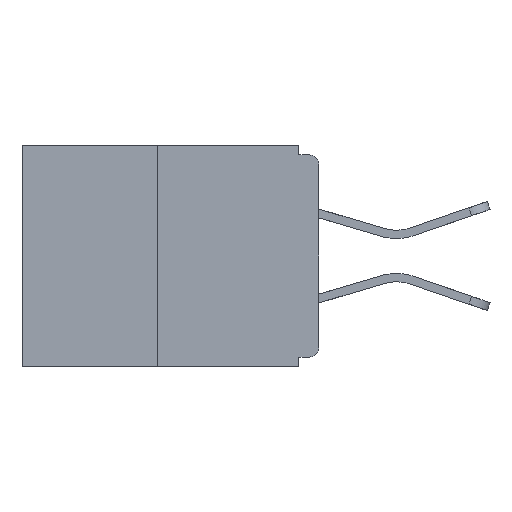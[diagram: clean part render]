
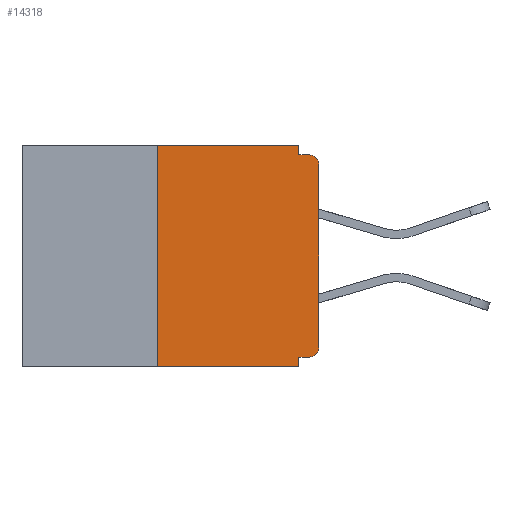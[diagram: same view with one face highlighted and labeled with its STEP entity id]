
A CAD part, left-side view. The second image highlights one B-rep face of the part: STEP entity #14318.
In plain terms, the highlighted planar face has unit normal (-1, 0, 0).
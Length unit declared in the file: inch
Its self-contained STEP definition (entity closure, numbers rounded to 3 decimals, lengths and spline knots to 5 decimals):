
#221 = PLANE ( 'NONE',  #11484 ) ;
#330 = DIRECTION ( 'NONE',  ( 0., 0., 1. ) ) ;
#594 = VERTEX_POINT ( 'NONE', #8248 ) ;
#719 = EDGE_LOOP ( 'NONE', ( #12575, #25406, #7802, #6723, #24492, #20611, #23564, #11362, #3248, #17616 ) ) ;
#834 = DIRECTION ( 'NONE',  ( 0., 0., -1. ) ) ;
#913 = CARTESIAN_POINT ( 'NONE',  ( 0., 0.031, -0.343 ) ) ;
#1100 = CARTESIAN_POINT ( 'NONE',  ( 0., 0., -0.03 ) ) ;
#1107 = DIRECTION ( 'NONE',  ( -1., 0., 0. ) ) ;
#1540 = AXIS2_PLACEMENT_3D ( 'NONE', #4196, #25913, #23711 ) ;
#1743 = FACE_OUTER_BOUND ( 'NONE', #719, .T. ) ;
#1822 = VERTEX_POINT ( 'NONE', #11964 ) ;
#2160 = DIRECTION ( 'NONE',  ( 0., 0., -1. ) ) ;
#2298 = VECTOR ( 'NONE', #2160, 39.37008 ) ;
#2478 = CARTESIAN_POINT ( 'NONE',  ( 0., 0., 0. ) ) ;
#3248 = ORIENTED_EDGE ( 'NONE', *, *, #22744, .F. ) ;
#3384 = VERTEX_POINT ( 'NONE', #913 ) ;
#3580 = VECTOR ( 'NONE', #10918, 39.37008 ) ;
#4196 = CARTESIAN_POINT ( 'NONE',  ( 0., 0.015, -0.03 ) ) ;
#4505 = CARTESIAN_POINT ( 'NONE',  ( 0., 0.25, 0. ) ) ;
#4918 = VECTOR ( 'NONE', #25838, 39.37008 ) ;
#5905 = VECTOR ( 'NONE', #13832, 39.37008 ) ;
#6216 = CARTESIAN_POINT ( 'NONE',  ( 0., 0.25, 0. ) ) ;
#6723 = ORIENTED_EDGE ( 'NONE', *, *, #21527, .F. ) ;
#7027 = VECTOR ( 'NONE', #12548, 39.37008 ) ;
#7417 = CARTESIAN_POINT ( 'NONE',  ( 0., 0., -0.015 ) ) ;
#7802 = ORIENTED_EDGE ( 'NONE', *, *, #17289, .T. ) ;
#8244 = VERTEX_POINT ( 'NONE', #6216 ) ;
#8248 = CARTESIAN_POINT ( 'NONE',  ( 0., 0.015, -0.015 ) ) ;
#9221 = CARTESIAN_POINT ( 'NONE',  ( 0., 0., -0.313 ) ) ;
#9269 = EDGE_CURVE ( 'NONE', #1822, #8244, #16037, .T. ) ;
#9451 = LINE ( 'NONE', #2478, #12472 ) ;
#10400 = VERTEX_POINT ( 'NONE', #1100 ) ;
#10918 = DIRECTION ( 'NONE',  ( 0., 0., -1. ) ) ;
#11362 = ORIENTED_EDGE ( 'NONE', *, *, #13192, .T. ) ;
#11373 = CARTESIAN_POINT ( 'NONE',  ( 0., 0.031, -0.015 ) ) ;
#11484 = AXIS2_PLACEMENT_3D ( 'NONE', #23931, #25879, #12940 ) ;
#11964 = CARTESIAN_POINT ( 'NONE',  ( 0., 0.25, -0.343 ) ) ;
#12164 = CARTESIAN_POINT ( 'NONE',  ( 0., 0.015, -0.328 ) ) ;
#12438 = AXIS2_PLACEMENT_3D ( 'NONE', #26858, #1107, #834 ) ;
#12472 = VECTOR ( 'NONE', #330, 39.37008 ) ;
#12548 = DIRECTION ( 'NONE',  ( 0., -1., 0. ) ) ;
#12575 = ORIENTED_EDGE ( 'NONE', *, *, #21542, .F. ) ;
#12905 = CARTESIAN_POINT ( 'NONE',  ( 0., 0.031, 0. ) ) ;
#12940 = DIRECTION ( 'NONE',  ( 0., 0., -1. ) ) ;
#12981 = DIRECTION ( 'NONE',  ( 0., -1., 0. ) ) ;
#13192 = EDGE_CURVE ( 'NONE', #10400, #594, #21598, .T. ) ;
#13521 = DIRECTION ( 'NONE',  ( 0., -1., 0. ) ) ;
#13662 = VECTOR ( 'NONE', #13521, 39.37008 ) ;
#13745 = LINE ( 'NONE', #23373, #2298 ) ;
#13832 = DIRECTION ( 'NONE',  ( 0., 1., 0. ) ) ;
#14118 = VERTEX_POINT ( 'NONE', #11373 ) ;
#14318 = ADVANCED_FACE ( 'NONE', ( #1743 ), #221, .F. ) ;
#15043 = LINE ( 'NONE', #12905, #3580 ) ;
#15318 = LINE ( 'NONE', #22411, #5905 ) ;
#16037 = LINE ( 'NONE', #4505, #4918 ) ;
#17093 = LINE ( 'NONE', #26173, #22148 ) ;
#17289 = EDGE_CURVE ( 'NONE', #1822, #3384, #17093, .T. ) ;
#17616 = ORIENTED_EDGE ( 'NONE', *, *, #26866, .F. ) ;
#19396 = VERTEX_POINT ( 'NONE', #9221 ) ;
#19577 = CARTESIAN_POINT ( 'NONE',  ( 0., 0.031, 0. ) ) ;
#20611 = ORIENTED_EDGE ( 'NONE', *, *, #26418, .T. ) ;
#21484 = CARTESIAN_POINT ( 'NONE',  ( 0., 0.46, 0. ) ) ;
#21527 = EDGE_CURVE ( 'NONE', #22442, #3384, #13745, .T. ) ;
#21542 = EDGE_CURVE ( 'NONE', #8244, #26188, #24510, .T. ) ;
#21598 = CIRCLE ( 'NONE', #1540, 0.015 ) ;
#22104 = LINE ( 'NONE', #7417, #13662 ) ;
#22148 = VECTOR ( 'NONE', #12981, 39.37008 ) ;
#22411 = CARTESIAN_POINT ( 'NONE',  ( 0., 0., -0.328 ) ) ;
#22442 = VERTEX_POINT ( 'NONE', #26619 ) ;
#22744 = EDGE_CURVE ( 'NONE', #14118, #594, #22104, .T. ) ;
#23373 = CARTESIAN_POINT ( 'NONE',  ( 0., 0.031, -0.343 ) ) ;
#23446 = EDGE_CURVE ( 'NONE', #24824, #22442, #15318, .T. ) ;
#23564 = ORIENTED_EDGE ( 'NONE', *, *, #25570, .T. ) ;
#23711 = DIRECTION ( 'NONE',  ( 0., 0., -1. ) ) ;
#23931 = CARTESIAN_POINT ( 'NONE',  ( 0., 0.46, 0. ) ) ;
#24492 = ORIENTED_EDGE ( 'NONE', *, *, #23446, .F. ) ;
#24510 = LINE ( 'NONE', #21484, #7027 ) ;
#24824 = VERTEX_POINT ( 'NONE', #12164 ) ;
#24828 = CIRCLE ( 'NONE', #12438, 0.015 ) ;
#25406 = ORIENTED_EDGE ( 'NONE', *, *, #9269, .F. ) ;
#25570 = EDGE_CURVE ( 'NONE', #19396, #10400, #9451, .T. ) ;
#25838 = DIRECTION ( 'NONE',  ( 0., 0., 1. ) ) ;
#25879 = DIRECTION ( 'NONE',  ( 1., 0., 0. ) ) ;
#25913 = DIRECTION ( 'NONE',  ( -1., 0., 0. ) ) ;
#26173 = CARTESIAN_POINT ( 'NONE',  ( 0., 0.46, -0.343 ) ) ;
#26188 = VERTEX_POINT ( 'NONE', #19577 ) ;
#26418 = EDGE_CURVE ( 'NONE', #24824, #19396, #24828, .T. ) ;
#26619 = CARTESIAN_POINT ( 'NONE',  ( 0., 0.031, -0.328 ) ) ;
#26858 = CARTESIAN_POINT ( 'NONE',  ( 0., 0.015, -0.313 ) ) ;
#26866 = EDGE_CURVE ( 'NONE', #26188, #14118, #15043, .T. ) ;
